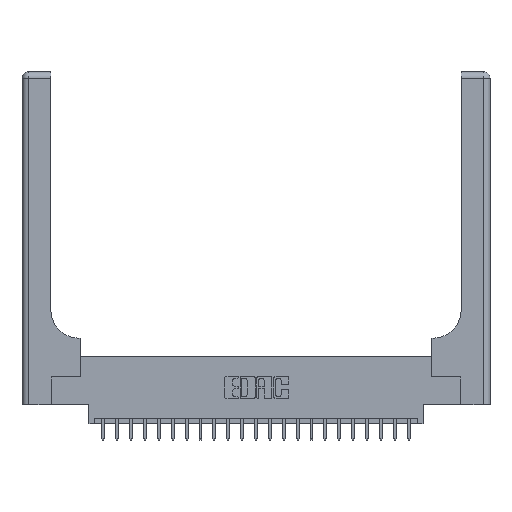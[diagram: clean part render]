
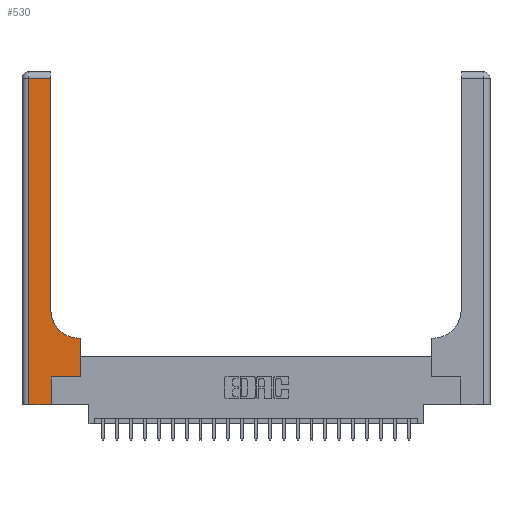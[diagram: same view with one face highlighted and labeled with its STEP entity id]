
A CAD part, top view. The second image highlights one B-rep face of the part: STEP entity #530.
In plain terms, the highlighted planar face has unit normal (0, 0, 1).
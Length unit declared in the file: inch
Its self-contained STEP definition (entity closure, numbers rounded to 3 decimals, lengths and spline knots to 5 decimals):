
#273 = CARTESIAN_POINT ( 'NONE',  ( 0.51, 0.85, 0.37 ) ) ;
#530 = ADVANCED_FACE ( 'NONE', ( #13543 ), #15084, .F. ) ;
#848 = DIRECTION ( 'NONE',  ( 1., 0., 0. ) ) ;
#1032 = DIRECTION ( 'NONE',  ( 0., 0., -1. ) ) ;
#1055 = ORIENTED_EDGE ( 'NONE', *, *, #17645, .T. ) ;
#1115 = CARTESIAN_POINT ( 'NONE',  ( 0.26, 3., 0.37 ) ) ;
#2147 = LINE ( 'NONE', #18433, #6853 ) ;
#2230 = VECTOR ( 'NONE', #5186, 39.37008 ) ;
#2254 = CARTESIAN_POINT ( 'NONE',  ( 0.265, 0.25, 0.37 ) ) ;
#2311 = CARTESIAN_POINT ( 'NONE',  ( 0., 2.94, 0.37 ) ) ;
#3093 = DIRECTION ( 'NONE',  ( 0., 1., 0. ) ) ;
#3539 = VERTEX_POINT ( 'NONE', #21484 ) ;
#3956 = EDGE_LOOP ( 'NONE', ( #1055, #16158, #6492, #19377, #21324, #7376, #18097, #14996, #5049 ) ) ;
#4374 = CARTESIAN_POINT ( 'NONE',  ( 0.51, 0.6, 0.37 ) ) ;
#4982 = VECTOR ( 'NONE', #6081, 39.37008 ) ;
#5049 = ORIENTED_EDGE ( 'NONE', *, *, #8614, .T. ) ;
#5186 = DIRECTION ( 'NONE',  ( 0., -1., 0. ) ) ;
#5361 = DIRECTION ( 'NONE',  ( -1., 0., 0. ) ) ;
#5715 = AXIS2_PLACEMENT_3D ( 'NONE', #17097, #1032, #19112 ) ;
#6081 = DIRECTION ( 'NONE',  ( -1., 0., 0. ) ) ;
#6492 = ORIENTED_EDGE ( 'NONE', *, *, #17020, .T. ) ;
#6853 = VECTOR ( 'NONE', #20090, 39.37008 ) ;
#7376 = ORIENTED_EDGE ( 'NONE', *, *, #16379, .T. ) ;
#7475 = DIRECTION ( 'NONE',  ( 0., 0., -1. ) ) ;
#8156 = VECTOR ( 'NONE', #5361, 39.37008 ) ;
#8209 = LINE ( 'NONE', #1115, #21120 ) ;
#8614 = EDGE_CURVE ( 'NONE', #17972, #18884, #10445, .T. ) ;
#8744 = VERTEX_POINT ( 'NONE', #13493 ) ;
#9937 = VECTOR ( 'NONE', #848, 39.37008 ) ;
#9982 = DIRECTION ( 'NONE',  ( 0., 1., 0. ) ) ;
#10072 = CARTESIAN_POINT ( 'NONE',  ( 0.528, 0.25, 0.37 ) ) ;
#10309 = LINE ( 'NONE', #14313, #22479 ) ;
#10445 = CIRCLE ( 'NONE', #13464, 0.25 ) ;
#10521 = VERTEX_POINT ( 'NONE', #2254 ) ;
#11413 = EDGE_CURVE ( 'NONE', #15464, #16421, #22042, .T. ) ;
#12059 = LINE ( 'NONE', #21157, #9937 ) ;
#12149 = CARTESIAN_POINT ( 'NONE',  ( 0.06, 3., 0.37 ) ) ;
#13464 = AXIS2_PLACEMENT_3D ( 'NONE', #273, #7475, #16111 ) ;
#13493 = CARTESIAN_POINT ( 'NONE',  ( 0.528, 0.25, 0.37 ) ) ;
#13543 = FACE_OUTER_BOUND ( 'NONE', #3956, .T. ) ;
#14313 = CARTESIAN_POINT ( 'NONE',  ( 0.265, 0., 0.37 ) ) ;
#14996 = ORIENTED_EDGE ( 'NONE', *, *, #22868, .T. ) ;
#15084 = PLANE ( 'NONE',  #5715 ) ;
#15384 = CARTESIAN_POINT ( 'NONE',  ( 0.06, 2.94, 0.37 ) ) ;
#15464 = VERTEX_POINT ( 'NONE', #20952 ) ;
#16110 = CARTESIAN_POINT ( 'NONE',  ( 0.528, 0.6, 0.37 ) ) ;
#16111 = DIRECTION ( 'NONE',  ( 1., 0., 0. ) ) ;
#16158 = ORIENTED_EDGE ( 'NONE', *, *, #11413, .T. ) ;
#16379 = EDGE_CURVE ( 'NONE', #10521, #8744, #12059, .T. ) ;
#16390 = EDGE_CURVE ( 'NONE', #8744, #17822, #19046, .T. ) ;
#16421 = VERTEX_POINT ( 'NONE', #15384 ) ;
#16952 = CARTESIAN_POINT ( 'NONE',  ( 0.06, 0., 0.37 ) ) ;
#17020 = EDGE_CURVE ( 'NONE', #16421, #21592, #21132, .T. ) ;
#17097 = CARTESIAN_POINT ( 'NONE',  ( 0., 3., 0.37 ) ) ;
#17645 = EDGE_CURVE ( 'NONE', #18884, #15464, #8209, .T. ) ;
#17822 = VERTEX_POINT ( 'NONE', #16110 ) ;
#17972 = VERTEX_POINT ( 'NONE', #4374 ) ;
#18097 = ORIENTED_EDGE ( 'NONE', *, *, #16390, .T. ) ;
#18433 = CARTESIAN_POINT ( 'NONE',  ( 0., 0., 0.37 ) ) ;
#18884 = VERTEX_POINT ( 'NONE', #18962 ) ;
#18962 = CARTESIAN_POINT ( 'NONE',  ( 0.26, 0.85, 0.37 ) ) ;
#18988 = VECTOR ( 'NONE', #22935, 39.37008 ) ;
#19046 = LINE ( 'NONE', #10072, #18988 ) ;
#19112 = DIRECTION ( 'NONE',  ( -1., 0., 0. ) ) ;
#19377 = ORIENTED_EDGE ( 'NONE', *, *, #19669, .T. ) ;
#19541 = LINE ( 'NONE', #19654, #8156 ) ;
#19654 = CARTESIAN_POINT ( 'NONE',  ( 0.26, 0.6, 0.37 ) ) ;
#19669 = EDGE_CURVE ( 'NONE', #21592, #3539, #2147, .T. ) ;
#20090 = DIRECTION ( 'NONE',  ( 1., 0., 0. ) ) ;
#20952 = CARTESIAN_POINT ( 'NONE',  ( 0.26, 2.94, 0.37 ) ) ;
#21120 = VECTOR ( 'NONE', #9982, 39.37008 ) ;
#21132 = LINE ( 'NONE', #12149, #2230 ) ;
#21157 = CARTESIAN_POINT ( 'NONE',  ( 0.265, 0.25, 0.37 ) ) ;
#21324 = ORIENTED_EDGE ( 'NONE', *, *, #23265, .T. ) ;
#21484 = CARTESIAN_POINT ( 'NONE',  ( 0.265, 0., 0.37 ) ) ;
#21592 = VERTEX_POINT ( 'NONE', #16952 ) ;
#22042 = LINE ( 'NONE', #2311, #4982 ) ;
#22479 = VECTOR ( 'NONE', #3093, 39.37008 ) ;
#22868 = EDGE_CURVE ( 'NONE', #17822, #17972, #19541, .T. ) ;
#22935 = DIRECTION ( 'NONE',  ( 0., 1., 0. ) ) ;
#23265 = EDGE_CURVE ( 'NONE', #3539, #10521, #10309, .T. ) ;
